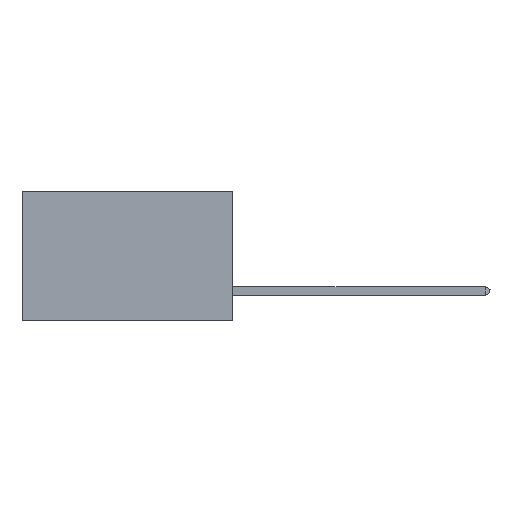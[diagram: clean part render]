
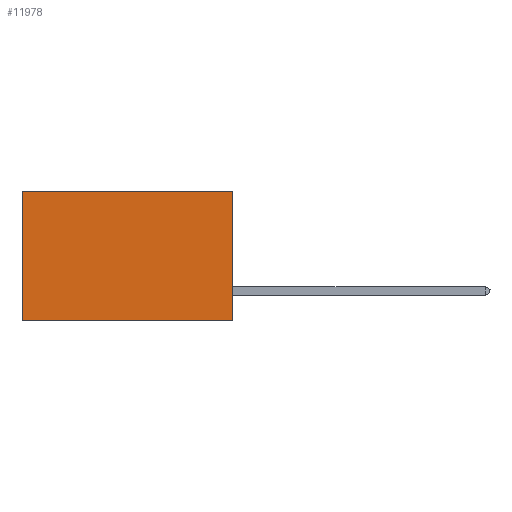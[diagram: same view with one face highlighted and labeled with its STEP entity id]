
A CAD part, left-side view. The second image highlights one B-rep face of the part: STEP entity #11978.
In plain terms, the highlighted planar face has unit normal (-1, 0, 0).
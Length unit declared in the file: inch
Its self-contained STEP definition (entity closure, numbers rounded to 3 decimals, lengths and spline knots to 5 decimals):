
#930 = FACE_OUTER_BOUND ( 'NONE', #12065, .T. ) ;
#1280 = ORIENTED_EDGE ( 'NONE', *, *, #13088, .T. ) ;
#3515 = CARTESIAN_POINT ( 'NONE',  ( 0.2875, 0., 0. ) ) ;
#5207 = CARTESIAN_POINT ( 'NONE',  ( 0.2875, 0.6, 0. ) ) ;
#5284 = AXIS2_PLACEMENT_3D ( 'NONE', #14419, #26826, #19472 ) ;
#5637 = CARTESIAN_POINT ( 'NONE',  ( 0.2875, 0., 0. ) ) ;
#6438 = CARTESIAN_POINT ( 'NONE',  ( 0.2875, 0.6, -0.37 ) ) ;
#6478 = VECTOR ( 'NONE', #18209, 39.37008 ) ;
#7574 = ORIENTED_EDGE ( 'NONE', *, *, #32292, .F. ) ;
#7654 = LINE ( 'NONE', #5637, #6478 ) ;
#8000 = ORIENTED_EDGE ( 'NONE', *, *, #9696, .F. ) ;
#8185 = VECTOR ( 'NONE', #28085, 39.37008 ) ;
#8598 = LINE ( 'NONE', #13008, #8185 ) ;
#9336 = PLANE ( 'NONE',  #5284 ) ;
#9696 = EDGE_CURVE ( 'NONE', #12735, #23869, #8598, .T. ) ;
#10793 = CARTESIAN_POINT ( 'NONE',  ( 0.2875, 0., 0. ) ) ;
#11978 = ADVANCED_FACE ( 'NONE', ( #930 ), #9336, .F. ) ;
#11986 = LINE ( 'NONE', #15510, #24367 ) ;
#12065 = EDGE_LOOP ( 'NONE', ( #20906, #8000, #7574, #1280 ) ) ;
#12735 = VERTEX_POINT ( 'NONE', #22889 ) ;
#13008 = CARTESIAN_POINT ( 'NONE',  ( 0.2875, 0., -0.37 ) ) ;
#13088 = EDGE_CURVE ( 'NONE', #30352, #20452, #22809, .T. ) ;
#14419 = CARTESIAN_POINT ( 'NONE',  ( 0.2875, 0., 0. ) ) ;
#15510 = CARTESIAN_POINT ( 'NONE',  ( 0.2875, 0.6, 0. ) ) ;
#17736 = EDGE_CURVE ( 'NONE', #20452, #23869, #11986, .T. ) ;
#18209 = DIRECTION ( 'NONE',  ( 0., 0., -1. ) ) ;
#19472 = DIRECTION ( 'NONE',  ( 0., 0., -1. ) ) ;
#20000 = VECTOR ( 'NONE', #21808, 39.37008 ) ;
#20452 = VERTEX_POINT ( 'NONE', #5207 ) ;
#20906 = ORIENTED_EDGE ( 'NONE', *, *, #17736, .T. ) ;
#21808 = DIRECTION ( 'NONE',  ( 0., 1., 0. ) ) ;
#22809 = LINE ( 'NONE', #3515, #20000 ) ;
#22838 = DIRECTION ( 'NONE',  ( 0., 0., -1. ) ) ;
#22889 = CARTESIAN_POINT ( 'NONE',  ( 0.2875, 0., -0.37 ) ) ;
#23869 = VERTEX_POINT ( 'NONE', #6438 ) ;
#24367 = VECTOR ( 'NONE', #22838, 39.37008 ) ;
#26826 = DIRECTION ( 'NONE',  ( 1., 0., 0. ) ) ;
#28085 = DIRECTION ( 'NONE',  ( 0., 1., 0. ) ) ;
#30352 = VERTEX_POINT ( 'NONE', #10793 ) ;
#32292 = EDGE_CURVE ( 'NONE', #30352, #12735, #7654, .T. ) ;
